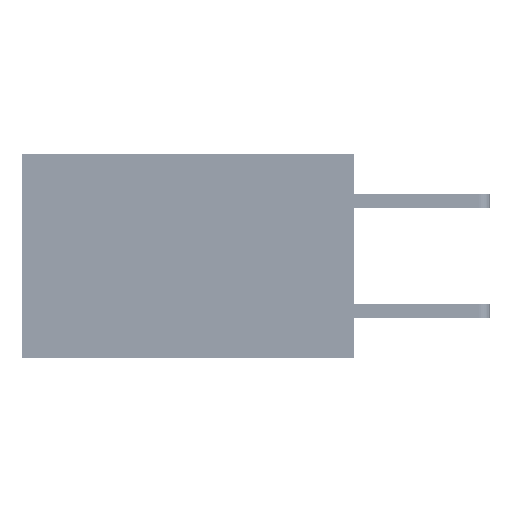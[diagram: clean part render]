
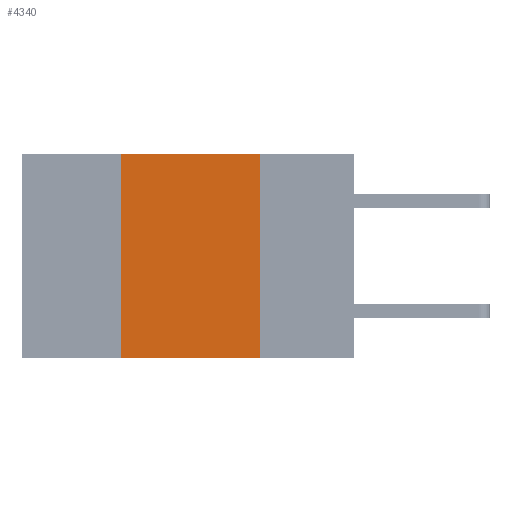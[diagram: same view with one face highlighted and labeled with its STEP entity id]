
A CAD part, left-side view. The second image highlights one B-rep face of the part: STEP entity #4340.
In plain terms, the highlighted planar face has unit normal (-1, 0, 0).
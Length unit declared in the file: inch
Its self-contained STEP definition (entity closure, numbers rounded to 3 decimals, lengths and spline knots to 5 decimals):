
#1148 = ORIENTED_EDGE ( 'NONE', *, *, #29718, .T. ) ;
#3565 = CARTESIAN_POINT ( 'NONE',  ( 0., 0.17, 0. ) ) ;
#3918 = VERTEX_POINT ( 'NONE', #36344 ) ;
#4124 = DIRECTION ( 'NONE',  ( 0., -1., 0. ) ) ;
#4340 = ADVANCED_FACE ( 'NONE', ( #10750 ), #41763, .F. ) ;
#4956 = EDGE_CURVE ( 'NONE', #24040, #36331, #24622, .T. ) ;
#5134 = LINE ( 'NONE', #27038, #19045 ) ;
#6877 = LINE ( 'NONE', #40530, #25436 ) ;
#9152 = VECTOR ( 'NONE', #28464, 39.37008 ) ;
#9787 = EDGE_CURVE ( 'NONE', #12082, #3918, #6877, .T. ) ;
#10750 = FACE_OUTER_BOUND ( 'NONE', #34258, .T. ) ;
#12082 = VERTEX_POINT ( 'NONE', #29783 ) ;
#14785 = AXIS2_PLACEMENT_3D ( 'NONE', #15953, #25750, #35284 ) ;
#15672 = CARTESIAN_POINT ( 'NONE',  ( 0., 0.6, -0.37 ) ) ;
#15953 = CARTESIAN_POINT ( 'NONE',  ( 0., 0.6, 0. ) ) ;
#17293 = DIRECTION ( 'NONE',  ( 0., 0., 1. ) ) ;
#18277 = CARTESIAN_POINT ( 'NONE',  ( 0., 0.17, -0.37 ) ) ;
#19045 = VECTOR ( 'NONE', #4124, 39.37008 ) ;
#20353 = EDGE_CURVE ( 'NONE', #3918, #24040, #5134, .T. ) ;
#24040 = VERTEX_POINT ( 'NONE', #3565 ) ;
#24622 = LINE ( 'NONE', #31633, #9152 ) ;
#25436 = VECTOR ( 'NONE', #17293, 39.37008 ) ;
#25750 = DIRECTION ( 'NONE',  ( 1., 0., 0. ) ) ;
#27038 = CARTESIAN_POINT ( 'NONE',  ( 0., 0.6, 0. ) ) ;
#27605 = ORIENTED_EDGE ( 'NONE', *, *, #9787, .F. ) ;
#28464 = DIRECTION ( 'NONE',  ( 0., 0., -1. ) ) ;
#29467 = LINE ( 'NONE', #15672, #32000 ) ;
#29718 = EDGE_CURVE ( 'NONE', #12082, #36331, #29467, .T. ) ;
#29783 = CARTESIAN_POINT ( 'NONE',  ( 0., 0.42, -0.37 ) ) ;
#29936 = ORIENTED_EDGE ( 'NONE', *, *, #4956, .F. ) ;
#31633 = CARTESIAN_POINT ( 'NONE',  ( 0., 0.17, 0. ) ) ;
#32000 = VECTOR ( 'NONE', #38466, 39.37008 ) ;
#34258 = EDGE_LOOP ( 'NONE', ( #29936, #34663, #27605, #1148 ) ) ;
#34663 = ORIENTED_EDGE ( 'NONE', *, *, #20353, .F. ) ;
#35284 = DIRECTION ( 'NONE',  ( 0., 0., -1. ) ) ;
#36331 = VERTEX_POINT ( 'NONE', #18277 ) ;
#36344 = CARTESIAN_POINT ( 'NONE',  ( 0., 0.42, 0. ) ) ;
#38466 = DIRECTION ( 'NONE',  ( 0., -1., 0. ) ) ;
#40530 = CARTESIAN_POINT ( 'NONE',  ( 0., 0.42, 0. ) ) ;
#41763 = PLANE ( 'NONE',  #14785 ) ;
